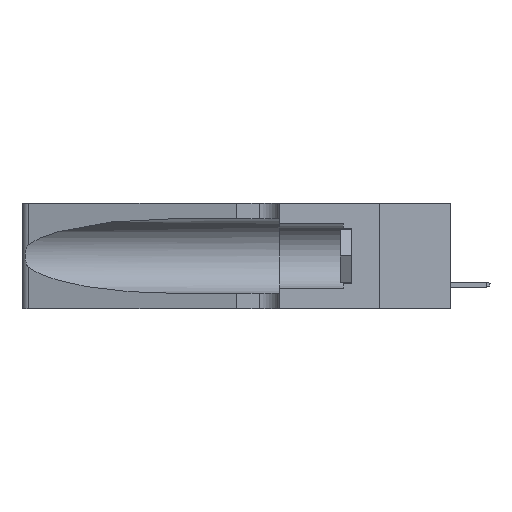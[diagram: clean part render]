
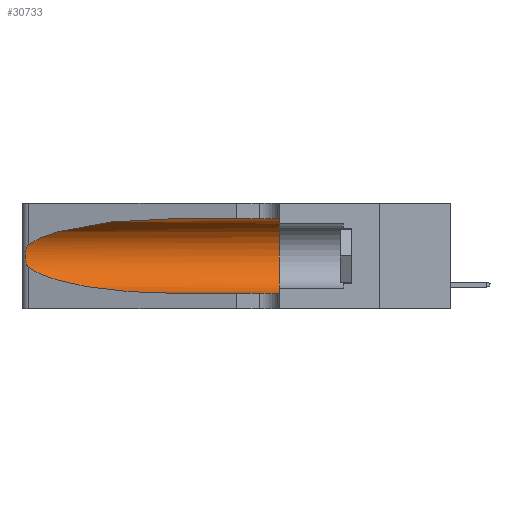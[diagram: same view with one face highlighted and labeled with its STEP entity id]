
A CAD part, left-side view. The second image highlights one B-rep face of the part: STEP entity #30733.
In plain terms, the highlighted cylindrical face has radius 3.308 mm (diameter 6.617 mm), a partial arc.
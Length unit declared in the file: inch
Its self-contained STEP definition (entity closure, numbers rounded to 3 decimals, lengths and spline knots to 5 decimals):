
#406 = VECTOR ( 'NONE', #7678, 39.37008 ) ;
#970 =( BOUNDED_CURVE ( )  B_SPLINE_CURVE ( 3, ( #15672, #22248, #9470, #28215 ),
 .UNSPECIFIED., .F., .F. ) 
 B_SPLINE_CURVE_WITH_KNOTS ( ( 4, 4 ),
 ( 1.5708, 2.84003 ),
 .UNSPECIFIED. ) 
 CURVE ( )  GEOMETRIC_REPRESENTATION_ITEM ( )  RATIONAL_B_SPLINE_CURVE ( ( 1., 0.87, 0.87, 1. ) ) 
 REPRESENTATION_ITEM ( '' )  );
#1129 = VERTEX_POINT ( 'NONE', #33829 ) ;
#2311 = CIRCLE ( 'NONE', #18732, 0.13025 ) ;
#2456 = DIRECTION ( 'NONE',  ( 0., 0., -1. ) ) ;
#4542 = CARTESIAN_POINT ( 'NONE',  ( 0.25639, 1.23184, 0.21858 ) ) ;
#4802 = EDGE_LOOP ( 'NONE', ( #8520, #14809, #27074, #17759, #27670, #13053 ) ) ;
#4804 = CARTESIAN_POINT ( 'NONE',  ( 0.18966, 0.96281, 0.05475 ) ) ;
#4937 = CARTESIAN_POINT ( 'NONE',  ( 0.25639, 1.23186, 0.15144 ) ) ;
#5854 = VERTEX_POINT ( 'NONE', #24422 ) ;
#5932 = DIRECTION ( 'NONE',  ( 0., -1., 0. ) ) ;
#7678 = DIRECTION ( 'NONE',  ( 0., -1., 0. ) ) ;
#7884 = CARTESIAN_POINT ( 'NONE',  ( 0.1305, 0.72297, 0.05475 ) ) ;
#8005 = CARTESIAN_POINT ( 'NONE',  ( 0.26075, 1.23896, 0.19203 ) ) ;
#8104 = CARTESIAN_POINT ( 'NONE',  ( 0.1305, 0.72297, 0.31525 ) ) ;
#8171 = VERTEX_POINT ( 'NONE', #8104 ) ;
#8520 = ORIENTED_EDGE ( 'NONE', *, *, #22159, .T. ) ;
#8871 = EDGE_CURVE ( 'NONE', #1129, #18237, #38758, .T. ) ;
#8994 = CYLINDRICAL_SURFACE ( 'NONE', #31620, 0.13025 ) ;
#9317 = VECTOR ( 'NONE', #23390, 39.37008 ) ;
#9470 = CARTESIAN_POINT ( 'NONE',  ( 0.2373, 1.15595, 0.28018 ) ) ;
#10973 = CARTESIAN_POINT ( 'NONE',  ( 0.1305, 1.61858, 0.31525 ) ) ;
#11111 = CARTESIAN_POINT ( 'NONE',  ( 0.25555, 1.22994, 0.2215 ) ) ;
#11300 = CARTESIAN_POINT ( 'NONE',  ( 0.25854, 1.2359, 0.20912 ) ) ;
#11508 = CARTESIAN_POINT ( 'NONE',  ( 0.25555, 1.22993, 0.14849 ) ) ;
#13053 = ORIENTED_EDGE ( 'NONE', *, *, #34241, .F. ) ;
#13883 = CARTESIAN_POINT ( 'NONE',  ( 0.25487, 1.22718, 0.14631 ) ) ;
#14412 = CARTESIAN_POINT ( 'NONE',  ( 0.26017, 1.23833, 0.17102 ) ) ;
#14615 = CARTESIAN_POINT ( 'NONE',  ( 0.25856, 1.23593, 0.16098 ) ) ;
#14809 = ORIENTED_EDGE ( 'NONE', *, *, #8871, .T. ) ;
#15472 = DIRECTION ( 'NONE',  ( 0., 1., 0. ) ) ;
#15672 = CARTESIAN_POINT ( 'NONE',  ( 0.1305, 0.72297, 0.31525 ) ) ;
#16511 = EDGE_CURVE ( 'NONE', #18237, #39420, #36171, .T. ) ;
#17209 = LINE ( 'NONE', #29578, #9317 ) ;
#17359 = EDGE_CURVE ( 'NONE', #39420, #25127, #17209, .T. ) ;
#17555 = LINE ( 'NONE', #10973, #406 ) ;
#17759 = ORIENTED_EDGE ( 'NONE', *, *, #17359, .T. ) ;
#18237 = VERTEX_POINT ( 'NONE', #34349 ) ;
#18732 = AXIS2_PLACEMENT_3D ( 'NONE', #19171, #15472, #28007 ) ;
#19171 = CARTESIAN_POINT ( 'NONE',  ( 0.1305, 0.35, 0.185 ) ) ;
#19269 = CARTESIAN_POINT ( 'NONE',  ( 0.1305, 0.72297, 0.05475 ) ) ;
#20586 = CARTESIAN_POINT ( 'NONE',  ( 0.25789, 1.23486, 0.15765 ) ) ;
#22122 = EDGE_CURVE ( 'NONE', #5854, #25127, #2311, .T. ) ;
#22159 = EDGE_CURVE ( 'NONE', #8171, #1129, #970, .T. ) ;
#22248 = CARTESIAN_POINT ( 'NONE',  ( 0.18966, 0.96281, 0.31525 ) ) ;
#22479 = CARTESIAN_POINT ( 'NONE',  ( 0.1305, 0.35, 0.05475 ) ) ;
#23390 = DIRECTION ( 'NONE',  ( 0., -1., 0. ) ) ;
#23664 = CARTESIAN_POINT ( 'NONE',  ( 0.25787, 1.23484, 0.2124 ) ) ;
#24422 = CARTESIAN_POINT ( 'NONE',  ( 0.1305, 0.35, 0.31525 ) ) ;
#25127 = VERTEX_POINT ( 'NONE', #22479 ) ;
#26625 = CARTESIAN_POINT ( 'NONE',  ( 0.2373, 1.15595, 0.08982 ) ) ;
#26965 = CARTESIAN_POINT ( 'NONE',  ( 0.25487, 1.22718, 0.14631 ) ) ;
#27074 = ORIENTED_EDGE ( 'NONE', *, *, #16511, .T. ) ;
#27670 = ORIENTED_EDGE ( 'NONE', *, *, #22122, .F. ) ;
#28007 = DIRECTION ( 'NONE',  ( 0., 0., 1. ) ) ;
#28215 = CARTESIAN_POINT ( 'NONE',  ( 0.25487, 1.22718, 0.22369 ) ) ;
#29578 = CARTESIAN_POINT ( 'NONE',  ( 0.1305, 1.61858, 0.05475 ) ) ;
#30733 = ADVANCED_FACE ( 'NONE', ( #33524 ), #8994, .F. ) ;
#31620 = AXIS2_PLACEMENT_3D ( 'NONE', #33723, #5932, #2456 ) ;
#33524 = FACE_OUTER_BOUND ( 'NONE', #4802, .T. ) ;
#33723 = CARTESIAN_POINT ( 'NONE',  ( 0.1305, 1.61858, 0.185 ) ) ;
#33829 = CARTESIAN_POINT ( 'NONE',  ( 0.25487, 1.22718, 0.22369 ) ) ;
#34241 = EDGE_CURVE ( 'NONE', #8171, #5854, #17555, .T. ) ;
#34349 = CARTESIAN_POINT ( 'NONE',  ( 0.25487, 1.22718, 0.14631 ) ) ;
#36171 =( BOUNDED_CURVE ( )  B_SPLINE_CURVE ( 3, ( #13883, #26625, #4804, #7884 ),
 .UNSPECIFIED., .F., .F. ) 
 B_SPLINE_CURVE_WITH_KNOTS ( ( 4, 4 ),
 ( 3.44316, 4.71239 ),
 .UNSPECIFIED. ) 
 CURVE ( )  GEOMETRIC_REPRESENTATION_ITEM ( )  RATIONAL_B_SPLINE_CURVE ( ( 1., 0.87, 0.87, 1. ) ) 
 REPRESENTATION_ITEM ( '' )  );
#38758 = B_SPLINE_CURVE_WITH_KNOTS ( 'NONE', 3,
 ( #39330, #11111, #4542, #23664, #11300, #39727, #8005, #39135, #14412, #14615, #20586, #4937, #11508, #26965 ),
 .UNSPECIFIED., .F., .F.,
 ( 4, 2, 2, 2, 2, 2, 4 ),
 ( 0., 0.00027, 0.00053, 0.00107, 0.0016, 0.00187, 0.00214 ),
 .UNSPECIFIED. ) ;
#39135 = CARTESIAN_POINT ( 'NONE',  ( 0.26075, 1.23896, 0.178 ) ) ;
#39330 = CARTESIAN_POINT ( 'NONE',  ( 0.25487, 1.22718, 0.22369 ) ) ;
#39420 = VERTEX_POINT ( 'NONE', #19269 ) ;
#39727 = CARTESIAN_POINT ( 'NONE',  ( 0.26018, 1.23835, 0.19895 ) ) ;
